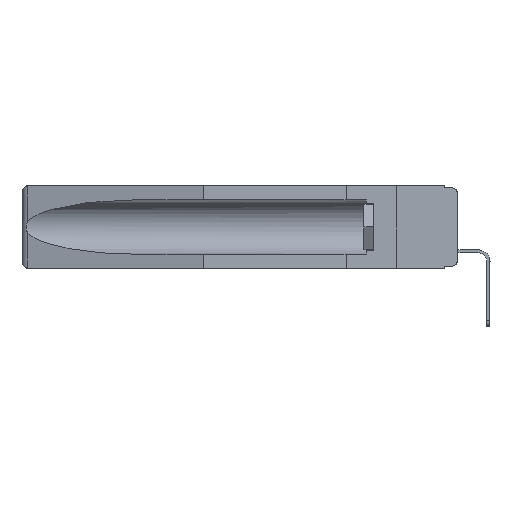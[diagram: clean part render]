
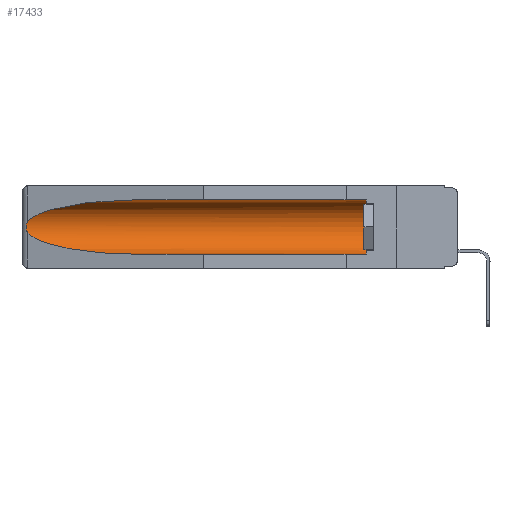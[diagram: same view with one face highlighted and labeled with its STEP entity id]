
A CAD part, left-side view. The second image highlights one B-rep face of the part: STEP entity #17433.
In plain terms, the highlighted cylindrical face has radius 2.857 mm (diameter 5.715 mm), a partial arc.
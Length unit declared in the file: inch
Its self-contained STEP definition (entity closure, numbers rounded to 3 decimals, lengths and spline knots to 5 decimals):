
#118 = CARTESIAN_POINT ( 'NONE',  ( 0.21114, 1.30732, -0.284 ) ) ;
#132 = EDGE_CURVE ( 'NONE', #8402, #3808, #14596, .T. ) ;
#251 = VERTEX_POINT ( 'NONE', #6221 ) ;
#436 = FACE_OUTER_BOUND ( 'NONE', #13413, .T. ) ;
#469 = CARTESIAN_POINT ( 'NONE',  ( 0.155, 1.07973, -0.059 ) ) ;
#1041 = LINE ( 'NONE', #9346, #14524 ) ;
#1369 = AXIS2_PLACEMENT_3D ( 'NONE', #4038, #11422, #10059 ) ;
#2593 = DIRECTION ( 'NONE',  ( 0., 1., 0. ) ) ;
#2772 = ORIENTED_EDGE ( 'NONE', *, *, #14296, .T. ) ;
#3232 = EDGE_CURVE ( 'NONE', #251, #13747, #12099, .T. ) ;
#3300 = CARTESIAN_POINT ( 'NONE',  ( 0.155, 1.07973, -0.059 ) ) ;
#3367 =( BOUNDED_CURVE ( )  B_SPLINE_CURVE ( 3, ( #3300, #6096, #4646, #8888 ),
 .UNSPECIFIED., .F., .F. ) 
 B_SPLINE_CURVE_WITH_KNOTS ( ( 4, 4 ),
 ( 4.71239, 6.08839 ),
 .UNSPECIFIED. ) 
 CURVE ( )  GEOMETRIC_REPRESENTATION_ITEM ( )  RATIONAL_B_SPLINE_CURVE ( ( 1., 0.848, 0.848, 1. ) ) 
 REPRESENTATION_ITEM ( '' )  );
#3542 = CARTESIAN_POINT ( 'NONE',  ( 0.26654, 1.53092, -0.15636 ) ) ;
#3667 = CARTESIAN_POINT ( 'NONE',  ( 0.26537, 1.52718, -0.14972 ) ) ;
#3808 = VERTEX_POINT ( 'NONE', #7272 ) ;
#4038 = CARTESIAN_POINT ( 'NONE',  ( 0.155, 0.126, -0.1715 ) ) ;
#4646 = CARTESIAN_POINT ( 'NONE',  ( 0.25451, 1.48313, -0.09465 ) ) ;
#4810 = CARTESIAN_POINT ( 'NONE',  ( 0.25451, 1.48313, -0.24835 ) ) ;
#4836 = LINE ( 'NONE', #15774, #16376 ) ;
#4961 = CARTESIAN_POINT ( 'NONE',  ( 0.2675, 1.53308, -0.17534 ) ) ;
#5188 = CARTESIAN_POINT ( 'NONE',  ( 0.26597, 1.52961, -0.15275 ) ) ;
#5492 = CARTESIAN_POINT ( 'NONE',  ( 0.155, -0.30754, -0.1715 ) ) ;
#5742 = VERTEX_POINT ( 'NONE', #469 ) ;
#5833 = EDGE_CURVE ( 'NONE', #8402, #15391, #4836, .T. ) ;
#6096 = CARTESIAN_POINT ( 'NONE',  ( 0.21114, 1.30732, -0.059 ) ) ;
#6221 = CARTESIAN_POINT ( 'NONE',  ( 0.26537, 1.52718, -0.14972 ) ) ;
#6347 = CARTESIAN_POINT ( 'NONE',  ( 0.26597, 1.5296, -0.19026 ) ) ;
#7272 = CARTESIAN_POINT ( 'NONE',  ( 0.155, 0.126, -0.059 ) ) ;
#7756 = CARTESIAN_POINT ( 'NONE',  ( 0.26537, 1.52718, -0.19328 ) ) ;
#7822 = CARTESIAN_POINT ( 'NONE',  ( 0.2673, 1.5327, -0.16383 ) ) ;
#7877 = CARTESIAN_POINT ( 'NONE',  ( 0.2673, 1.53269, -0.17917 ) ) ;
#8402 = VERTEX_POINT ( 'NONE', #15318 ) ;
#8888 = CARTESIAN_POINT ( 'NONE',  ( 0.26537, 1.52718, -0.14972 ) ) ;
#8935 = CARTESIAN_POINT ( 'NONE',  ( 0.26537, 1.52718, -0.19328 ) ) ;
#9063 =( BOUNDED_CURVE ( )  B_SPLINE_CURVE ( 3, ( #8935, #4810, #118, #13462 ),
 .UNSPECIFIED., .F., .T. ) 
 B_SPLINE_CURVE_WITH_KNOTS ( ( 4, 4 ),
 ( 0.1948, 1.5708 ),
 .UNSPECIFIED. ) 
 CURVE ( )  GEOMETRIC_REPRESENTATION_ITEM ( )  RATIONAL_B_SPLINE_CURVE ( ( 1., 0.848, 0.848, 1. ) ) 
 REPRESENTATION_ITEM ( '' )  );
#9099 = ORIENTED_EDGE ( 'NONE', *, *, #9438, .T. ) ;
#9346 = CARTESIAN_POINT ( 'NONE',  ( 0.155, -0.30754, -0.059 ) ) ;
#9438 = EDGE_CURVE ( 'NONE', #3808, #5742, #1041, .T. ) ;
#9807 = DIRECTION ( 'NONE',  ( 0., 1., 0. ) ) ;
#10059 = DIRECTION ( 'NONE',  ( 0., 0., 1. ) ) ;
#10172 = ORIENTED_EDGE ( 'NONE', *, *, #5833, .F. ) ;
#10688 = ORIENTED_EDGE ( 'NONE', *, *, #3232, .T. ) ;
#11422 = DIRECTION ( 'NONE',  ( 0., -1., 0. ) ) ;
#11625 = CARTESIAN_POINT ( 'NONE',  ( 0.26537, 1.52718, -0.19328 ) ) ;
#11650 = AXIS2_PLACEMENT_3D ( 'NONE', #5492, #9807, #12338 ) ;
#12099 = B_SPLINE_CURVE_WITH_KNOTS ( 'NONE', 3,
 ( #3667, #5188, #3542, #7822, #13419, #4961, #7877, #14683, #6347, #7756 ),
 .UNSPECIFIED., .F., .F.,
 ( 4, 2, 2, 2, 4 ),
 ( 0., 0.00029, 0.00058, 0.00087, 0.00117 ),
 .UNSPECIFIED. ) ;
#12170 = CYLINDRICAL_SURFACE ( 'NONE', #11650, 0.1125 ) ;
#12338 = DIRECTION ( 'NONE',  ( 0., 0., 1. ) ) ;
#12480 = CARTESIAN_POINT ( 'NONE',  ( 0.155, 1.07973, -0.284 ) ) ;
#13374 = ORIENTED_EDGE ( 'NONE', *, *, #132, .T. ) ;
#13413 = EDGE_LOOP ( 'NONE', ( #15020, #10688, #2772, #10172, #13374, #9099 ) ) ;
#13419 = CARTESIAN_POINT ( 'NONE',  ( 0.2675, 1.53308, -0.16763 ) ) ;
#13462 = CARTESIAN_POINT ( 'NONE',  ( 0.155, 1.07973, -0.284 ) ) ;
#13747 = VERTEX_POINT ( 'NONE', #11625 ) ;
#14238 = DIRECTION ( 'NONE',  ( 0., 1., 0. ) ) ;
#14296 = EDGE_CURVE ( 'NONE', #13747, #15391, #9063, .T. ) ;
#14524 = VECTOR ( 'NONE', #2593, 39.37008 ) ;
#14596 = CIRCLE ( 'NONE', #1369, 0.1125 ) ;
#14683 = CARTESIAN_POINT ( 'NONE',  ( 0.26655, 1.53094, -0.18657 ) ) ;
#15020 = ORIENTED_EDGE ( 'NONE', *, *, #17635, .T. ) ;
#15318 = CARTESIAN_POINT ( 'NONE',  ( 0.155, 0.126, -0.284 ) ) ;
#15391 = VERTEX_POINT ( 'NONE', #12480 ) ;
#15774 = CARTESIAN_POINT ( 'NONE',  ( 0.155, -0.30754, -0.284 ) ) ;
#16376 = VECTOR ( 'NONE', #14238, 39.37008 ) ;
#17433 = ADVANCED_FACE ( 'NONE', ( #436 ), #12170, .F. ) ;
#17635 = EDGE_CURVE ( 'NONE', #5742, #251, #3367, .T. ) ;
